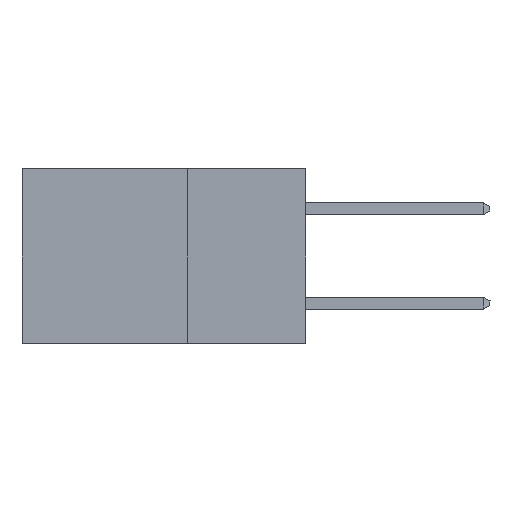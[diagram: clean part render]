
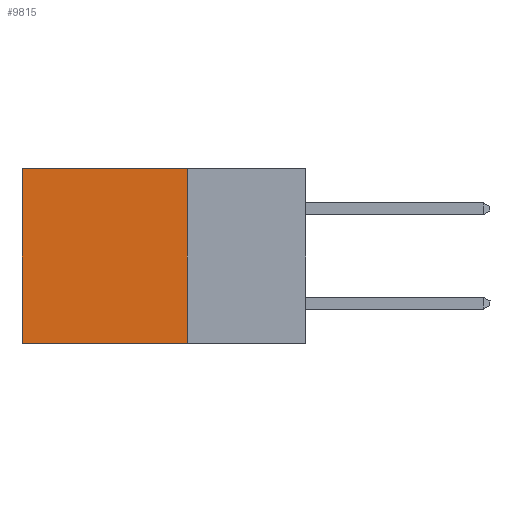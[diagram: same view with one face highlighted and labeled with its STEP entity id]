
A CAD part, left-side view. The second image highlights one B-rep face of the part: STEP entity #9815.
In plain terms, the highlighted planar face has unit normal (-1, 0, 0).
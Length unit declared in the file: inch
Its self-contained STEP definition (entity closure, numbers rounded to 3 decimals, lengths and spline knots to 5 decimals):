
#592 = FACE_OUTER_BOUND ( 'NONE', #3372, .T. ) ;
#1541 = CARTESIAN_POINT ( 'NONE',  ( 0.2615, 0.6, -0.37 ) ) ;
#1673 = DIRECTION ( 'NONE',  ( 1., 0., 0. ) ) ;
#2899 = EDGE_CURVE ( 'NONE', #15470, #21269, #5344, .T. ) ;
#3372 = EDGE_LOOP ( 'NONE', ( #7023, #6635, #22744, #5590 ) ) ;
#5344 = LINE ( 'NONE', #1541, #15075 ) ;
#5515 = CARTESIAN_POINT ( 'NONE',  ( 0.2615, 0.6, -0.37 ) ) ;
#5590 = ORIENTED_EDGE ( 'NONE', *, *, #6114, .T. ) ;
#5781 = LINE ( 'NONE', #18623, #20616 ) ;
#6114 = EDGE_CURVE ( 'NONE', #8159, #15470, #5781, .T. ) ;
#6635 = ORIENTED_EDGE ( 'NONE', *, *, #19084, .F. ) ;
#7023 = ORIENTED_EDGE ( 'NONE', *, *, #2899, .T. ) ;
#7032 = CARTESIAN_POINT ( 'NONE',  ( 0.2615, 0.25, 0. ) ) ;
#7438 = VERTEX_POINT ( 'NONE', #22165 ) ;
#8159 = VERTEX_POINT ( 'NONE', #7032 ) ;
#8439 = VECTOR ( 'NONE', #11871, 39.37008 ) ;
#9053 = LINE ( 'NONE', #17571, #8439 ) ;
#9574 = CARTESIAN_POINT ( 'NONE',  ( 0.2615, 0.25, -0.37 ) ) ;
#9815 = ADVANCED_FACE ( 'NONE', ( #592 ), #13477, .F. ) ;
#10168 = VECTOR ( 'NONE', #21927, 39.37008 ) ;
#11871 = DIRECTION ( 'NONE',  ( 0., 0., -1. ) ) ;
#12377 = CARTESIAN_POINT ( 'NONE',  ( 0.2615, 0.6, 0. ) ) ;
#13477 = PLANE ( 'NONE',  #20038 ) ;
#14156 = CARTESIAN_POINT ( 'NONE',  ( 0.2615, 0.25, -0.37 ) ) ;
#15075 = VECTOR ( 'NONE', #15257, 39.37008 ) ;
#15257 = DIRECTION ( 'NONE',  ( 0., 0., -1. ) ) ;
#15386 = DIRECTION ( 'NONE',  ( 0., 0., -1. ) ) ;
#15470 = VERTEX_POINT ( 'NONE', #12377 ) ;
#17571 = CARTESIAN_POINT ( 'NONE',  ( 0.2615, 0.25, -0.37 ) ) ;
#18623 = CARTESIAN_POINT ( 'NONE',  ( 0.2615, 0.25, 0. ) ) ;
#19084 = EDGE_CURVE ( 'NONE', #7438, #21269, #20401, .T. ) ;
#20038 = AXIS2_PLACEMENT_3D ( 'NONE', #9574, #1673, #15386 ) ;
#20401 = LINE ( 'NONE', #14156, #10168 ) ;
#20616 = VECTOR ( 'NONE', #24412, 39.37008 ) ;
#21269 = VERTEX_POINT ( 'NONE', #5515 ) ;
#21927 = DIRECTION ( 'NONE',  ( 0., 1., 0. ) ) ;
#22165 = CARTESIAN_POINT ( 'NONE',  ( 0.2615, 0.25, -0.37 ) ) ;
#22744 = ORIENTED_EDGE ( 'NONE', *, *, #25080, .F. ) ;
#24412 = DIRECTION ( 'NONE',  ( 0., 1., 0. ) ) ;
#25080 = EDGE_CURVE ( 'NONE', #8159, #7438, #9053, .T. ) ;
